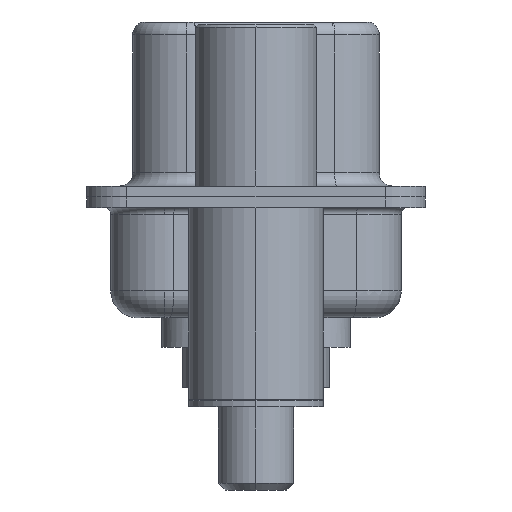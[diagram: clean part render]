
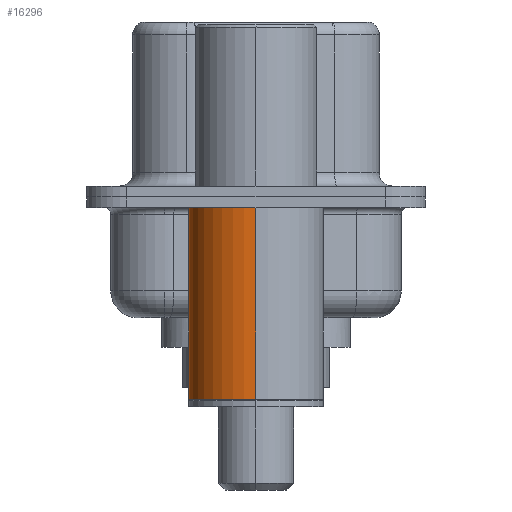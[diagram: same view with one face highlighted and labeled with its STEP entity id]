
A CAD part, left-side view. The second image highlights one B-rep face of the part: STEP entity #16296.
In plain terms, the highlighted cylindrical face has radius 2.5 mm (diameter 5 mm), a partial arc.
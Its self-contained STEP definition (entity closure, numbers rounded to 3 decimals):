
#212 = VERTEX_POINT ( 'NONE', #11969 ) ;
#354 = DIRECTION ( 'NONE',  ( 0., 0., 1. ) ) ;
#447 = VERTEX_POINT ( 'NONE', #11495 ) ;
#497 = AXIS2_PLACEMENT_3D ( 'NONE', #5423, #1365, #13900 ) ;
#1365 = DIRECTION ( 'NONE',  ( 0., 0., 1. ) ) ;
#1918 = VERTEX_POINT ( 'NONE', #14853 ) ;
#3811 = CARTESIAN_POINT ( 'NONE',  ( -2.5, 0., 0.581 ) ) ;
#4644 = EDGE_CURVE ( 'NONE', #1918, #11089, #4788, .T. ) ;
#4788 = LINE ( 'NONE', #16677, #13425 ) ;
#5364 = DIRECTION ( 'NONE',  ( 0., 0., 1. ) ) ;
#5417 = VECTOR ( 'NONE', #5364, 1000. ) ;
#5423 = CARTESIAN_POINT ( 'NONE',  ( 0., 0., 0.581 ) ) ;
#5812 = EDGE_LOOP ( 'NONE', ( #15554, #7871, #7995, #10027 ) ) ;
#6530 = AXIS2_PLACEMENT_3D ( 'NONE', #16357, #16539, #8045 ) ;
#6938 = AXIS2_PLACEMENT_3D ( 'NONE', #8410, #354, #7020 ) ;
#7020 = DIRECTION ( 'NONE',  ( 1., 0., 0. ) ) ;
#7255 = CARTESIAN_POINT ( 'NONE',  ( 2.5, 0., -0.4 ) ) ;
#7871 = ORIENTED_EDGE ( 'NONE', *, *, #17154, .T. ) ;
#7995 = ORIENTED_EDGE ( 'NONE', *, *, #15283, .F. ) ;
#8045 = DIRECTION ( 'NONE',  ( 1., 0., 0. ) ) ;
#8410 = CARTESIAN_POINT ( 'NONE',  ( 0., 0., -7.525 ) ) ;
#10027 = ORIENTED_EDGE ( 'NONE', *, *, #4644, .F. ) ;
#11089 = VERTEX_POINT ( 'NONE', #7255 ) ;
#11134 = EDGE_CURVE ( 'NONE', #1918, #212, #14206, .T. ) ;
#11495 = CARTESIAN_POINT ( 'NONE',  ( -2.5, 0., -0.4 ) ) ;
#11948 = CYLINDRICAL_SURFACE ( 'NONE', #497, 2.5 ) ;
#11969 = CARTESIAN_POINT ( 'NONE',  ( -2.5, 0., -7.525 ) ) ;
#13051 = CIRCLE ( 'NONE', #6530, 2.5 ) ;
#13425 = VECTOR ( 'NONE', #16566, 1000. ) ;
#13900 = DIRECTION ( 'NONE',  ( 1., 0., 0. ) ) ;
#14206 = CIRCLE ( 'NONE', #6938, 2.5 ) ;
#14759 = FACE_OUTER_BOUND ( 'NONE', #5812, .T. ) ;
#14853 = CARTESIAN_POINT ( 'NONE',  ( 2.5, 0., -7.525 ) ) ;
#15283 = EDGE_CURVE ( 'NONE', #11089, #447, #13051, .T. ) ;
#15554 = ORIENTED_EDGE ( 'NONE', *, *, #11134, .T. ) ;
#16296 = ADVANCED_FACE ( 'NONE', ( #14759 ), #11948, .T. ) ;
#16357 = CARTESIAN_POINT ( 'NONE',  ( 0., 0., -0.4 ) ) ;
#16495 = LINE ( 'NONE', #3811, #5417 ) ;
#16539 = DIRECTION ( 'NONE',  ( 0., 0., 1. ) ) ;
#16566 = DIRECTION ( 'NONE',  ( 0., 0., 1. ) ) ;
#16677 = CARTESIAN_POINT ( 'NONE',  ( 2.5, 0., 0.581 ) ) ;
#17154 = EDGE_CURVE ( 'NONE', #212, #447, #16495, .T. ) ;
